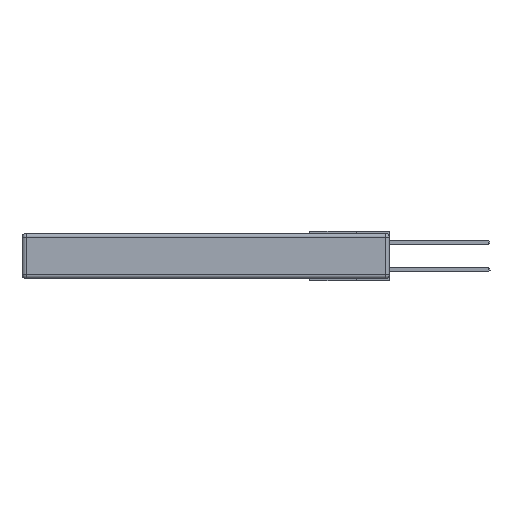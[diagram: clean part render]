
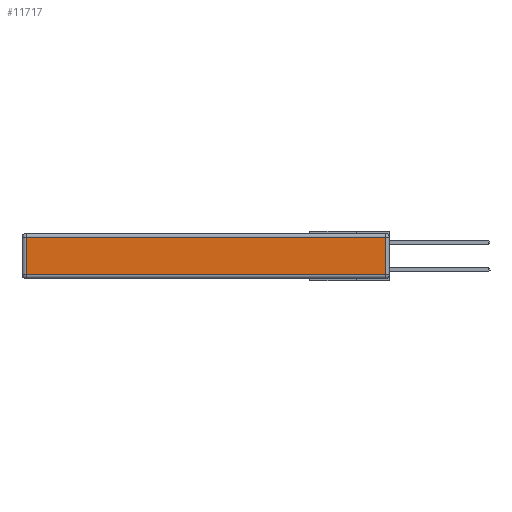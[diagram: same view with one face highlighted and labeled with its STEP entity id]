
A CAD part, left-side view. The second image highlights one B-rep face of the part: STEP entity #11717.
In plain terms, the highlighted planar face has unit normal (-1, 0, 0).
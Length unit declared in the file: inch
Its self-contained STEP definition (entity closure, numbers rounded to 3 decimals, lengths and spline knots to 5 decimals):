
#442 = DIRECTION ( 'NONE',  ( 0., 0., -1. ) ) ;
#484 = CARTESIAN_POINT ( 'NONE',  ( 0., 2.72, -0.03 ) ) ;
#696 = VECTOR ( 'NONE', #3580, 39.37008 ) ;
#878 = PLANE ( 'NONE',  #7625 ) ;
#1027 = DIRECTION ( 'NONE',  ( 0., -1., 0. ) ) ;
#1087 = DIRECTION ( 'NONE',  ( 0., 0., 1. ) ) ;
#1098 = VERTEX_POINT ( 'NONE', #4574 ) ;
#1539 = CARTESIAN_POINT ( 'NONE',  ( 0., 2.72, -0.313 ) ) ;
#1770 = LINE ( 'NONE', #9276, #17379 ) ;
#3089 = VECTOR ( 'NONE', #1027, 39.37008 ) ;
#3236 = LINE ( 'NONE', #10450, #696 ) ;
#3580 = DIRECTION ( 'NONE',  ( 0., 1., 0. ) ) ;
#3712 = LINE ( 'NONE', #16035, #3089 ) ;
#3727 = DIRECTION ( 'NONE',  ( -1., 0., 0. ) ) ;
#3770 = ORIENTED_EDGE ( 'NONE', *, *, #13290, .T. ) ;
#3794 = DIRECTION ( 'NONE',  ( 0., 0., 1. ) ) ;
#4574 = CARTESIAN_POINT ( 'NONE',  ( 0., 0.03, -0.03 ) ) ;
#6359 = EDGE_CURVE ( 'NONE', #8011, #12450, #7136, .T. ) ;
#7136 = LINE ( 'NONE', #7148, #16590 ) ;
#7148 = CARTESIAN_POINT ( 'NONE',  ( 0., 2.72, -0.343 ) ) ;
#7625 = AXIS2_PLACEMENT_3D ( 'NONE', #14543, #3727, #3794 ) ;
#8011 = VERTEX_POINT ( 'NONE', #484 ) ;
#8524 = EDGE_CURVE ( 'NONE', #1098, #8011, #3236, .T. ) ;
#8857 = VERTEX_POINT ( 'NONE', #14799 ) ;
#9276 = CARTESIAN_POINT ( 'NONE',  ( 0., 0.03, -0.343 ) ) ;
#10450 = CARTESIAN_POINT ( 'NONE',  ( 0., 2.75, -0.03 ) ) ;
#10808 = EDGE_LOOP ( 'NONE', ( #12725, #3770, #12885, #17016 ) ) ;
#11717 = ADVANCED_FACE ( 'NONE', ( #14494 ), #878, .T. ) ;
#12450 = VERTEX_POINT ( 'NONE', #1539 ) ;
#12725 = ORIENTED_EDGE ( 'NONE', *, *, #17381, .T. ) ;
#12885 = ORIENTED_EDGE ( 'NONE', *, *, #8524, .T. ) ;
#13290 = EDGE_CURVE ( 'NONE', #8857, #1098, #1770, .T. ) ;
#14494 = FACE_OUTER_BOUND ( 'NONE', #10808, .T. ) ;
#14543 = CARTESIAN_POINT ( 'NONE',  ( 0., 0., -0.343 ) ) ;
#14799 = CARTESIAN_POINT ( 'NONE',  ( 0., 0.03, -0.313 ) ) ;
#16035 = CARTESIAN_POINT ( 'NONE',  ( 0., 0., -0.313 ) ) ;
#16590 = VECTOR ( 'NONE', #442, 39.37008 ) ;
#17016 = ORIENTED_EDGE ( 'NONE', *, *, #6359, .T. ) ;
#17379 = VECTOR ( 'NONE', #1087, 39.37008 ) ;
#17381 = EDGE_CURVE ( 'NONE', #12450, #8857, #3712, .T. ) ;
